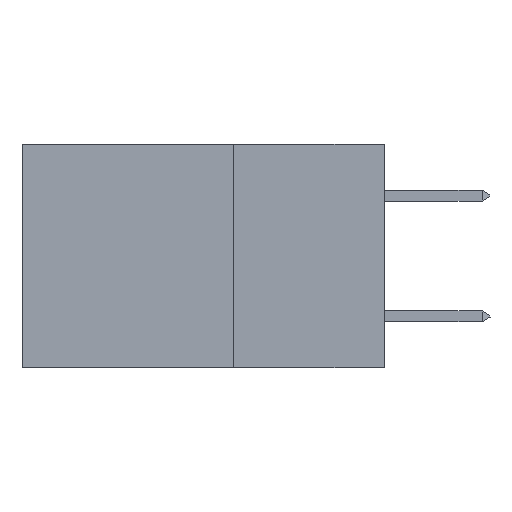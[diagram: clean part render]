
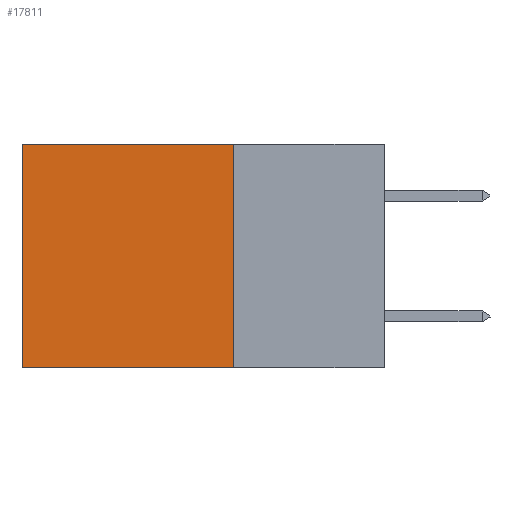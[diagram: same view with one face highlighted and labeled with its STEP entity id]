
A CAD part, left-side view. The second image highlights one B-rep face of the part: STEP entity #17811.
In plain terms, the highlighted planar face has unit normal (-1, 0, 0).
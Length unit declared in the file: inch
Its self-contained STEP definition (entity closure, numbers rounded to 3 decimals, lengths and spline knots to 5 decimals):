
#2453 = EDGE_LOOP ( 'NONE', ( #41652, #27873, #39559, #41986 ) ) ;
#3508 = VERTEX_POINT ( 'NONE', #17661 ) ;
#3622 = VECTOR ( 'NONE', #21511, 39.37008 ) ;
#3651 = VECTOR ( 'NONE', #20525, 39.37008 ) ;
#4499 = CARTESIAN_POINT ( 'NONE',  ( 0.2875, 0.25, 0. ) ) ;
#5521 = EDGE_CURVE ( 'NONE', #5558, #3508, #6424, .T. ) ;
#5558 = VERTEX_POINT ( 'NONE', #26888 ) ;
#5974 = DIRECTION ( 'NONE',  ( 1., 0., 0. ) ) ;
#6424 = LINE ( 'NONE', #11090, #34883 ) ;
#8227 = DIRECTION ( 'NONE',  ( 0., 1., 0. ) ) ;
#8251 = VECTOR ( 'NONE', #20946, 39.37008 ) ;
#8468 = EDGE_CURVE ( 'NONE', #35723, #3508, #17463, .T. ) ;
#9425 = AXIS2_PLACEMENT_3D ( 'NONE', #32258, #5974, #38617 ) ;
#11090 = CARTESIAN_POINT ( 'NONE',  ( 0.2875, 0.25, -0.37 ) ) ;
#12699 = FACE_OUTER_BOUND ( 'NONE', #2453, .T. ) ;
#17463 = LINE ( 'NONE', #30939, #8251 ) ;
#17661 = CARTESIAN_POINT ( 'NONE',  ( 0.2875, 0.6, -0.37 ) ) ;
#17811 = ADVANCED_FACE ( 'NONE', ( #12699 ), #35303, .F. ) ;
#18014 = CARTESIAN_POINT ( 'NONE',  ( 0.2875, 0.25, 0. ) ) ;
#19660 = LINE ( 'NONE', #4499, #3651 ) ;
#20525 = DIRECTION ( 'NONE',  ( 0., 1., 0. ) ) ;
#20946 = DIRECTION ( 'NONE',  ( 0., 0., -1. ) ) ;
#21511 = DIRECTION ( 'NONE',  ( 0., 0., -1. ) ) ;
#25920 = EDGE_CURVE ( 'NONE', #26603, #5558, #40878, .T. ) ;
#26603 = VERTEX_POINT ( 'NONE', #29194 ) ;
#26888 = CARTESIAN_POINT ( 'NONE',  ( 0.2875, 0.25, -0.37 ) ) ;
#27873 = ORIENTED_EDGE ( 'NONE', *, *, #5521, .F. ) ;
#29194 = CARTESIAN_POINT ( 'NONE',  ( 0.2875, 0.25, 0. ) ) ;
#30939 = CARTESIAN_POINT ( 'NONE',  ( 0.2875, 0.6, 0. ) ) ;
#32258 = CARTESIAN_POINT ( 'NONE',  ( 0.2875, 0.25, 0. ) ) ;
#34883 = VECTOR ( 'NONE', #8227, 39.37008 ) ;
#35303 = PLANE ( 'NONE',  #9425 ) ;
#35723 = VERTEX_POINT ( 'NONE', #42417 ) ;
#38617 = DIRECTION ( 'NONE',  ( 0., 0., -1. ) ) ;
#39559 = ORIENTED_EDGE ( 'NONE', *, *, #25920, .F. ) ;
#40878 = LINE ( 'NONE', #18014, #3622 ) ;
#41652 = ORIENTED_EDGE ( 'NONE', *, *, #8468, .T. ) ;
#41986 = ORIENTED_EDGE ( 'NONE', *, *, #42562, .T. ) ;
#42417 = CARTESIAN_POINT ( 'NONE',  ( 0.2875, 0.6, 0. ) ) ;
#42562 = EDGE_CURVE ( 'NONE', #26603, #35723, #19660, .T. ) ;
